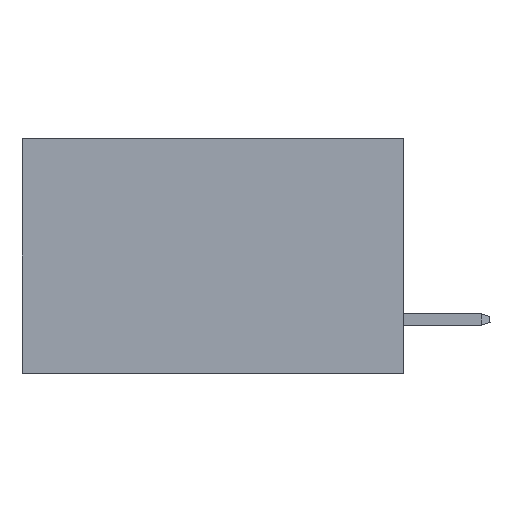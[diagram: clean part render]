
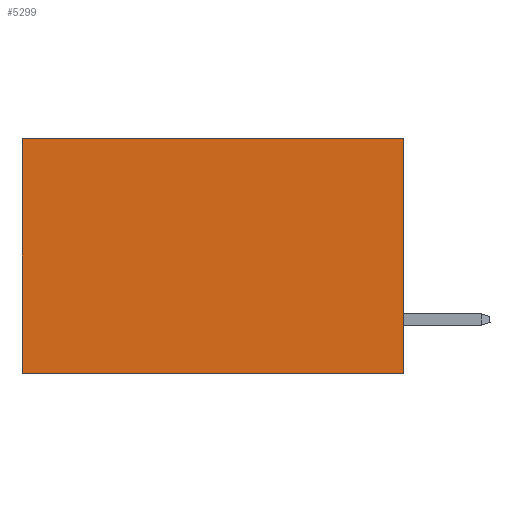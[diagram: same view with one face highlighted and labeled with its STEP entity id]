
A CAD part, left-side view. The second image highlights one B-rep face of the part: STEP entity #5299.
In plain terms, the highlighted planar face has unit normal (-1, 0, 0).
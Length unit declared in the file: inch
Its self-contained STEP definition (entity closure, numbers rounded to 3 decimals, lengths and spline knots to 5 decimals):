
#467 = DIRECTION ( 'NONE',  ( 0., 0., -1. ) ) ;
#1929 = PLANE ( 'NONE',  #35844 ) ;
#2010 = CARTESIAN_POINT ( 'NONE',  ( 0.2875, 0.6, 0. ) ) ;
#4808 = EDGE_LOOP ( 'NONE', ( #6667, #24945, #14992, #29582 ) ) ;
#5299 = ADVANCED_FACE ( 'NONE', ( #39621 ), #1929, .F. ) ;
#6659 = DIRECTION ( 'NONE',  ( 0., 0., -1. ) ) ;
#6667 = ORIENTED_EDGE ( 'NONE', *, *, #31697, .T. ) ;
#9226 = CARTESIAN_POINT ( 'NONE',  ( 0.2875, 0., -0.37 ) ) ;
#9242 = LINE ( 'NONE', #2010, #22879 ) ;
#10341 = LINE ( 'NONE', #25700, #21469 ) ;
#13636 = VERTEX_POINT ( 'NONE', #23773 ) ;
#14992 = ORIENTED_EDGE ( 'NONE', *, *, #27857, .F. ) ;
#17476 = CARTESIAN_POINT ( 'NONE',  ( 0.2875, 0., 0. ) ) ;
#17529 = EDGE_CURVE ( 'NONE', #36777, #13636, #27419, .T. ) ;
#17800 = DIRECTION ( 'NONE',  ( 1., 0., 0. ) ) ;
#18733 = CARTESIAN_POINT ( 'NONE',  ( 0.2875, 0., 0. ) ) ;
#21133 = VERTEX_POINT ( 'NONE', #46460 ) ;
#21403 = DIRECTION ( 'NONE',  ( 0., 1., 0. ) ) ;
#21469 = VECTOR ( 'NONE', #21403, 39.37008 ) ;
#22879 = VECTOR ( 'NONE', #27714, 39.37008 ) ;
#23773 = CARTESIAN_POINT ( 'NONE',  ( 0.2875, 0.6, -0.37 ) ) ;
#24679 = LINE ( 'NONE', #17476, #35935 ) ;
#24945 = ORIENTED_EDGE ( 'NONE', *, *, #17529, .F. ) ;
#25700 = CARTESIAN_POINT ( 'NONE',  ( 0.2875, 0., 0. ) ) ;
#27419 = LINE ( 'NONE', #31973, #33719 ) ;
#27714 = DIRECTION ( 'NONE',  ( 0., 0., -1. ) ) ;
#27857 = EDGE_CURVE ( 'NONE', #21133, #36777, #24679, .T. ) ;
#29582 = ORIENTED_EDGE ( 'NONE', *, *, #38599, .T. ) ;
#31697 = EDGE_CURVE ( 'NONE', #31721, #13636, #9242, .T. ) ;
#31721 = VERTEX_POINT ( 'NONE', #46212 ) ;
#31973 = CARTESIAN_POINT ( 'NONE',  ( 0.2875, 0., -0.37 ) ) ;
#33719 = VECTOR ( 'NONE', #46619, 39.37008 ) ;
#35844 = AXIS2_PLACEMENT_3D ( 'NONE', #18733, #17800, #467 ) ;
#35935 = VECTOR ( 'NONE', #6659, 39.37008 ) ;
#36777 = VERTEX_POINT ( 'NONE', #9226 ) ;
#38599 = EDGE_CURVE ( 'NONE', #21133, #31721, #10341, .T. ) ;
#39621 = FACE_OUTER_BOUND ( 'NONE', #4808, .T. ) ;
#46212 = CARTESIAN_POINT ( 'NONE',  ( 0.2875, 0.6, 0. ) ) ;
#46460 = CARTESIAN_POINT ( 'NONE',  ( 0.2875, 0., 0. ) ) ;
#46619 = DIRECTION ( 'NONE',  ( 0., 1., 0. ) ) ;
